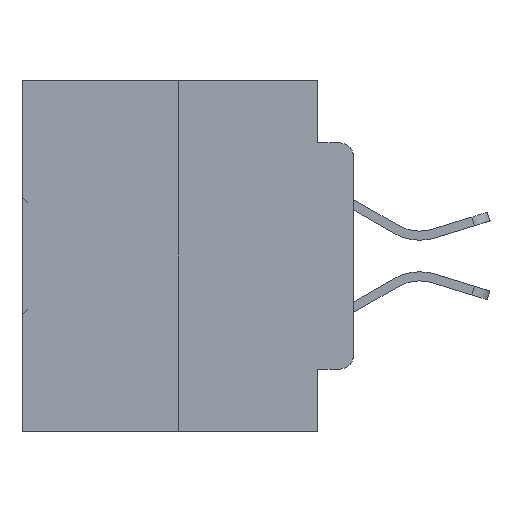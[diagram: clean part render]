
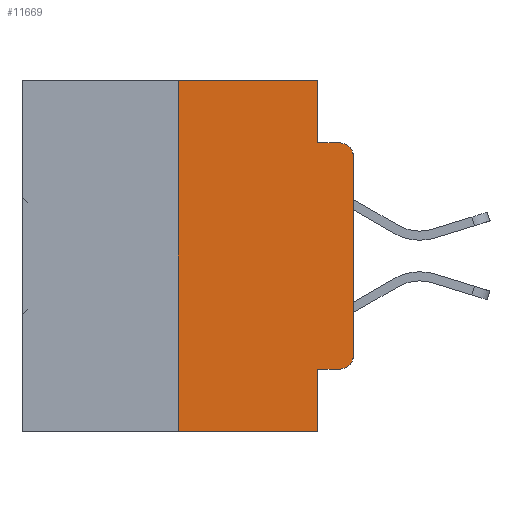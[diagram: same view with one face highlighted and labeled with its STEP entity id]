
A CAD part, left-side view. The second image highlights one B-rep face of the part: STEP entity #11669.
In plain terms, the highlighted planar face has unit normal (-1, 0, 0).
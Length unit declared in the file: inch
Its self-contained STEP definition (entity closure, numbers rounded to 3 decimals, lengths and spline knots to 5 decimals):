
#921 = CARTESIAN_POINT ( 'NONE',  ( 0., 0.25, 0. ) ) ;
#1361 = CARTESIAN_POINT ( 'NONE',  ( 0., 0.25, 0. ) ) ;
#1470 = VERTEX_POINT ( 'NONE', #3821 ) ;
#1566 = DIRECTION ( 'NONE',  ( 1., 0., 0. ) ) ;
#2878 = ORIENTED_EDGE ( 'NONE', *, *, #21142, .T. ) ;
#3015 = VERTEX_POINT ( 'NONE', #14350 ) ;
#3298 = ORIENTED_EDGE ( 'NONE', *, *, #10434, .F. ) ;
#3468 = CARTESIAN_POINT ( 'NONE',  ( 0., 0.473, -0.5 ) ) ;
#3821 = CARTESIAN_POINT ( 'NONE',  ( 0., 0.051, 0. ) ) ;
#4260 = CARTESIAN_POINT ( 'NONE',  ( 0., 0., -0.1085 ) ) ;
#4769 = VERTEX_POINT ( 'NONE', #16663 ) ;
#5235 = CARTESIAN_POINT ( 'NONE',  ( 0., 0.02, -0.0885 ) ) ;
#5888 = DIRECTION ( 'NONE',  ( 0., 0., -1. ) ) ;
#6741 = CARTESIAN_POINT ( 'NONE',  ( 0., 0., 0. ) ) ;
#6748 = VECTOR ( 'NONE', #30612, 39.37008 ) ;
#7905 = EDGE_CURVE ( 'NONE', #23667, #23644, #32531, .T. ) ;
#8873 = CIRCLE ( 'NONE', #34328, 0.02 ) ;
#9454 = VERTEX_POINT ( 'NONE', #26837 ) ;
#10297 = DIRECTION ( 'NONE',  ( 0., -1., 0. ) ) ;
#10434 = EDGE_CURVE ( 'NONE', #3015, #26931, #23706, .T. ) ;
#10646 = VECTOR ( 'NONE', #10297, 39.37008 ) ;
#11669 = ADVANCED_FACE ( 'NONE', ( #15974 ), #15584, .F. ) ;
#12164 = EDGE_CURVE ( 'NONE', #9454, #34814, #19767, .T. ) ;
#12978 = CARTESIAN_POINT ( 'NONE',  ( 0., 0.473, 0. ) ) ;
#13885 = ORIENTED_EDGE ( 'NONE', *, *, #12164, .T. ) ;
#14066 = CIRCLE ( 'NONE', #18248, 0.02 ) ;
#14282 = CARTESIAN_POINT ( 'NONE',  ( 0., 0.02, -0.3915 ) ) ;
#14350 = CARTESIAN_POINT ( 'NONE',  ( 0., 0.25, -0.5 ) ) ;
#15176 = DIRECTION ( 'NONE',  ( 0., 0., 1. ) ) ;
#15498 = EDGE_CURVE ( 'NONE', #23667, #34418, #26322, .T. ) ;
#15584 = PLANE ( 'NONE',  #30904 ) ;
#15974 = FACE_OUTER_BOUND ( 'NONE', #17607, .T. ) ;
#16190 = DIRECTION ( 'NONE',  ( -1., 0., 0. ) ) ;
#16436 = ORIENTED_EDGE ( 'NONE', *, *, #28886, .F. ) ;
#16663 = CARTESIAN_POINT ( 'NONE',  ( 0., 0.051, -0.0885 ) ) ;
#17058 = DIRECTION ( 'NONE',  ( 0., 0., -1. ) ) ;
#17598 = CARTESIAN_POINT ( 'NONE',  ( 0., 0.051, -0.4115 ) ) ;
#17607 = EDGE_LOOP ( 'NONE', ( #13885, #20096, #31773, #26376, #16436, #3298, #34448, #22381, #31448, #2878 ) ) ;
#18248 = AXIS2_PLACEMENT_3D ( 'NONE', #14282, #33485, #17058 ) ;
#18726 = CARTESIAN_POINT ( 'NONE',  ( 0., 0.051, -0.0885 ) ) ;
#19363 = EDGE_CURVE ( 'NONE', #1470, #4769, #29628, .T. ) ;
#19459 = LINE ( 'NONE', #18726, #34078 ) ;
#19767 = LINE ( 'NONE', #6741, #26149 ) ;
#20096 = ORIENTED_EDGE ( 'NONE', *, *, #27611, .T. ) ;
#20200 = CARTESIAN_POINT ( 'NONE',  ( 0., 0.02, -0.4115 ) ) ;
#20437 = DIRECTION ( 'NONE',  ( 0., 0., 1. ) ) ;
#21055 = DIRECTION ( 'NONE',  ( 0., 0., -1. ) ) ;
#21142 = EDGE_CURVE ( 'NONE', #23644, #9454, #14066, .T. ) ;
#21314 = CARTESIAN_POINT ( 'NONE',  ( 0., 0.051, -0.4115 ) ) ;
#21455 = DIRECTION ( 'NONE',  ( 0., -1., 0. ) ) ;
#22381 = ORIENTED_EDGE ( 'NONE', *, *, #15498, .F. ) ;
#22432 = CARTESIAN_POINT ( 'NONE',  ( 0., 0.051, 0. ) ) ;
#22871 = VERTEX_POINT ( 'NONE', #5235 ) ;
#23644 = VERTEX_POINT ( 'NONE', #20200 ) ;
#23667 = VERTEX_POINT ( 'NONE', #17598 ) ;
#23706 = LINE ( 'NONE', #921, #31051 ) ;
#24601 = EDGE_CURVE ( 'NONE', #4769, #22871, #19459, .T. ) ;
#25602 = DIRECTION ( 'NONE',  ( 0., -1., 0. ) ) ;
#26149 = VECTOR ( 'NONE', #15176, 39.37008 ) ;
#26322 = LINE ( 'NONE', #22432, #27192 ) ;
#26376 = ORIENTED_EDGE ( 'NONE', *, *, #19363, .F. ) ;
#26837 = CARTESIAN_POINT ( 'NONE',  ( 0., 0., -0.3915 ) ) ;
#26931 = VERTEX_POINT ( 'NONE', #1361 ) ;
#27192 = VECTOR ( 'NONE', #5888, 39.37008 ) ;
#27296 = EDGE_CURVE ( 'NONE', #3015, #34418, #27380, .T. ) ;
#27338 = VECTOR ( 'NONE', #34914, 39.37008 ) ;
#27380 = LINE ( 'NONE', #3468, #33874 ) ;
#27611 = EDGE_CURVE ( 'NONE', #34814, #22871, #8873, .T. ) ;
#28886 = EDGE_CURVE ( 'NONE', #26931, #1470, #35536, .T. ) ;
#29628 = LINE ( 'NONE', #33288, #6748 ) ;
#30612 = DIRECTION ( 'NONE',  ( 0., 0., -1. ) ) ;
#30904 = AXIS2_PLACEMENT_3D ( 'NONE', #34747, #1566, #21055 ) ;
#31051 = VECTOR ( 'NONE', #20437, 39.37008 ) ;
#31448 = ORIENTED_EDGE ( 'NONE', *, *, #7905, .T. ) ;
#31773 = ORIENTED_EDGE ( 'NONE', *, *, #24601, .F. ) ;
#32531 = LINE ( 'NONE', #21314, #10646 ) ;
#32598 = CARTESIAN_POINT ( 'NONE',  ( 0., 0.02, -0.1085 ) ) ;
#33288 = CARTESIAN_POINT ( 'NONE',  ( 0., 0.051, 0. ) ) ;
#33485 = DIRECTION ( 'NONE',  ( -1., 0., 0. ) ) ;
#33874 = VECTOR ( 'NONE', #25602, 39.37008 ) ;
#34078 = VECTOR ( 'NONE', #21455, 39.37008 ) ;
#34328 = AXIS2_PLACEMENT_3D ( 'NONE', #32598, #16190, #35348 ) ;
#34418 = VERTEX_POINT ( 'NONE', #35691 ) ;
#34448 = ORIENTED_EDGE ( 'NONE', *, *, #27296, .T. ) ;
#34747 = CARTESIAN_POINT ( 'NONE',  ( 0., 0.473, 0. ) ) ;
#34814 = VERTEX_POINT ( 'NONE', #4260 ) ;
#34914 = DIRECTION ( 'NONE',  ( 0., -1., 0. ) ) ;
#35348 = DIRECTION ( 'NONE',  ( 0., 0., -1. ) ) ;
#35536 = LINE ( 'NONE', #12978, #27338 ) ;
#35691 = CARTESIAN_POINT ( 'NONE',  ( 0., 0.051, -0.5 ) ) ;
